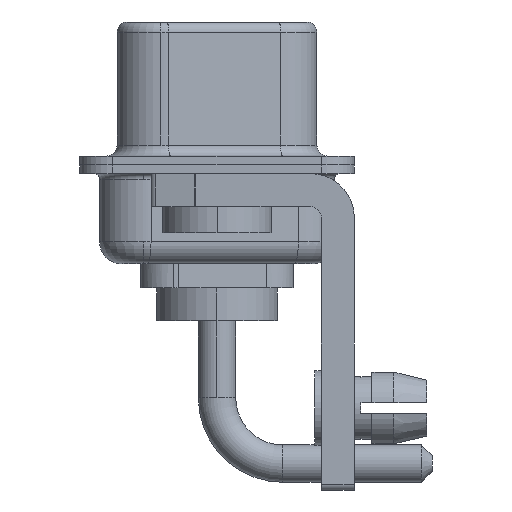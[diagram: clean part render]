
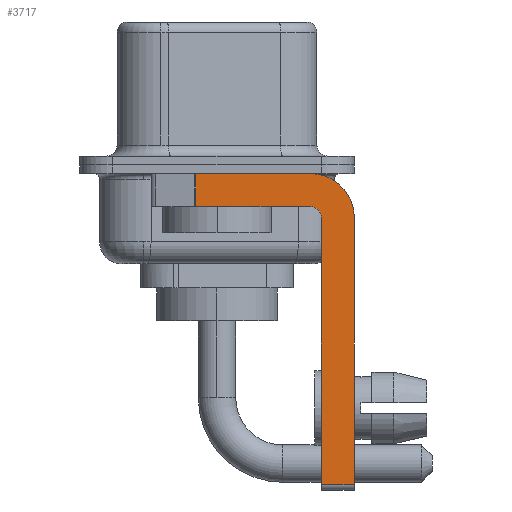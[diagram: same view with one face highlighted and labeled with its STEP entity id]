
A CAD part, left-side view. The second image highlights one B-rep face of the part: STEP entity #3717.
In plain terms, the highlighted planar face has unit normal (-1, 0, 0).
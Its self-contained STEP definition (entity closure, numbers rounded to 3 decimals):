
#267 = DIRECTION ( 'NONE',  ( -1., 0., 0. ) ) ;
#838 = EDGE_CURVE ( 'NONE', #13086, #16265, #4883, .T. ) ;
#930 = LINE ( 'NONE', #18216, #14920 ) ;
#1714 = CIRCLE ( 'NONE', #13766, 0.5 ) ;
#2065 = VECTOR ( 'NONE', #3217, 1000. ) ;
#2250 = ORIENTED_EDGE ( 'NONE', *, *, #2760, .T. ) ;
#2532 = FACE_OUTER_BOUND ( 'NONE', #9871, .T. ) ;
#2760 = EDGE_CURVE ( 'NONE', #15563, #18201, #6917, .T. ) ;
#2939 = DIRECTION ( 'NONE',  ( 1., 0., 0. ) ) ;
#3006 = ORIENTED_EDGE ( 'NONE', *, *, #13674, .F. ) ;
#3217 = DIRECTION ( 'NONE',  ( 0., 0., 1. ) ) ;
#3614 = EDGE_CURVE ( 'NONE', #13580, #5342, #1714, .T. ) ;
#3717 = ADVANCED_FACE ( 'NONE', ( #2532 ), #6785, .F. ) ;
#4260 = DIRECTION ( 'NONE',  ( 0., 0., -1. ) ) ;
#4441 = CARTESIAN_POINT ( 'NONE',  ( -2.9, -4.25, -2.4 ) ) ;
#4515 = LINE ( 'NONE', #11790, #8121 ) ;
#4543 = DIRECTION ( 'NONE',  ( 0., 0., -1. ) ) ;
#4883 = LINE ( 'NONE', #10639, #13854 ) ;
#5269 = CARTESIAN_POINT ( 'NONE',  ( -2.9, -4.25, -2.4 ) ) ;
#5279 = DIRECTION ( 'NONE',  ( 0., 1., 0. ) ) ;
#5342 = VERTEX_POINT ( 'NONE', #8347 ) ;
#5431 = VECTOR ( 'NONE', #4543, 1000. ) ;
#5594 = DIRECTION ( 'NONE',  ( 0., -1., 0. ) ) ;
#6719 = EDGE_CURVE ( 'NONE', #15563, #13580, #13311, .T. ) ;
#6762 = ORIENTED_EDGE ( 'NONE', *, *, #8042, .F. ) ;
#6785 = PLANE ( 'NONE',  #9928 ) ;
#6917 = LINE ( 'NONE', #9748, #15058 ) ;
#7166 = EDGE_CURVE ( 'NONE', #13086, #9261, #4515, .T. ) ;
#8042 = EDGE_CURVE ( 'NONE', #15326, #18201, #16238, .T. ) ;
#8121 = VECTOR ( 'NONE', #13108, 1000. ) ;
#8284 = DIRECTION ( 'NONE',  ( 0., 0., -1. ) ) ;
#8347 = CARTESIAN_POINT ( 'NONE',  ( -2.9, -4.25, -1.9 ) ) ;
#8685 = ORIENTED_EDGE ( 'NONE', *, *, #13321, .F. ) ;
#9261 = VERTEX_POINT ( 'NONE', #10528 ) ;
#9509 = DIRECTION ( 'NONE',  ( 1., 0., 0. ) ) ;
#9748 = CARTESIAN_POINT ( 'NONE',  ( -2.9, -4.25, -14.55 ) ) ;
#9871 = EDGE_LOOP ( 'NONE', ( #13110, #14826, #3006, #11975, #9882, #2250, #6762, #8685 ) ) ;
#9882 = ORIENTED_EDGE ( 'NONE', *, *, #6719, .F. ) ;
#9928 = AXIS2_PLACEMENT_3D ( 'NONE', #5269, #9509, #8284 ) ;
#10472 = CARTESIAN_POINT ( 'NONE',  ( -2.9, -4.25, -2.4 ) ) ;
#10528 = CARTESIAN_POINT ( 'NONE',  ( -2.9, -4.25, -0.4 ) ) ;
#10639 = CARTESIAN_POINT ( 'NONE',  ( -2.9, 0.978, -1.9 ) ) ;
#11583 = CIRCLE ( 'NONE', #18204, 2. ) ;
#11790 = CARTESIAN_POINT ( 'NONE',  ( -2.9, 3., -0.4 ) ) ;
#11975 = ORIENTED_EDGE ( 'NONE', *, *, #3614, .F. ) ;
#13086 = VERTEX_POINT ( 'NONE', #16362 ) ;
#13108 = DIRECTION ( 'NONE',  ( 0., -1., 0. ) ) ;
#13110 = ORIENTED_EDGE ( 'NONE', *, *, #7166, .F. ) ;
#13311 = LINE ( 'NONE', #14938, #2065 ) ;
#13315 = CARTESIAN_POINT ( 'NONE',  ( -2.9, -6.25, -2.4 ) ) ;
#13321 = EDGE_CURVE ( 'NONE', #9261, #15326, #11583, .T. ) ;
#13396 = DIRECTION ( 'NONE',  ( 0., 0., 1. ) ) ;
#13580 = VERTEX_POINT ( 'NONE', #16612 ) ;
#13674 = EDGE_CURVE ( 'NONE', #5342, #16265, #930, .T. ) ;
#13766 = AXIS2_PLACEMENT_3D ( 'NONE', #10472, #267, #13396 ) ;
#13854 = VECTOR ( 'NONE', #16395, 1000. ) ;
#14826 = ORIENTED_EDGE ( 'NONE', *, *, #838, .T. ) ;
#14920 = VECTOR ( 'NONE', #5279, 1000. ) ;
#14938 = CARTESIAN_POINT ( 'NONE',  ( -2.9, -4.75, -14.8 ) ) ;
#15058 = VECTOR ( 'NONE', #5594, 1000. ) ;
#15109 = CARTESIAN_POINT ( 'NONE',  ( -2.9, -6.25, -2.4 ) ) ;
#15310 = CARTESIAN_POINT ( 'NONE',  ( -2.9, -6.25, -14.55 ) ) ;
#15326 = VERTEX_POINT ( 'NONE', #15109 ) ;
#15523 = CARTESIAN_POINT ( 'NONE',  ( -2.9, 0.978, -1.9 ) ) ;
#15563 = VERTEX_POINT ( 'NONE', #17246 ) ;
#16238 = LINE ( 'NONE', #13315, #5431 ) ;
#16265 = VERTEX_POINT ( 'NONE', #15523 ) ;
#16362 = CARTESIAN_POINT ( 'NONE',  ( -2.9, 0.978, -0.4 ) ) ;
#16395 = DIRECTION ( 'NONE',  ( 0., 0., -1. ) ) ;
#16612 = CARTESIAN_POINT ( 'NONE',  ( -2.9, -4.75, -2.4 ) ) ;
#17246 = CARTESIAN_POINT ( 'NONE',  ( -2.9, -4.75, -14.55 ) ) ;
#18201 = VERTEX_POINT ( 'NONE', #15310 ) ;
#18204 = AXIS2_PLACEMENT_3D ( 'NONE', #4441, #2939, #4260 ) ;
#18216 = CARTESIAN_POINT ( 'NONE',  ( -2.9, -4.25, -1.9 ) ) ;
